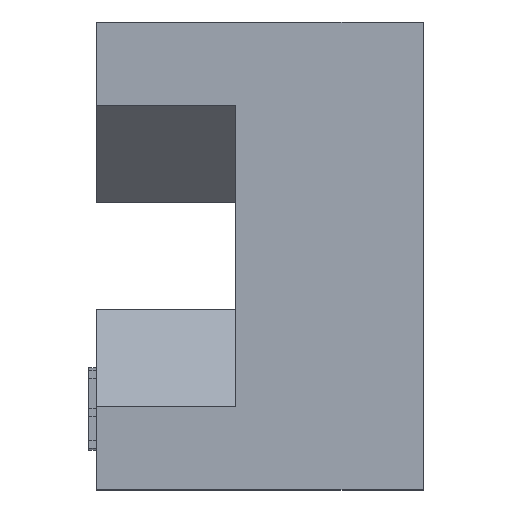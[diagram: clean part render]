
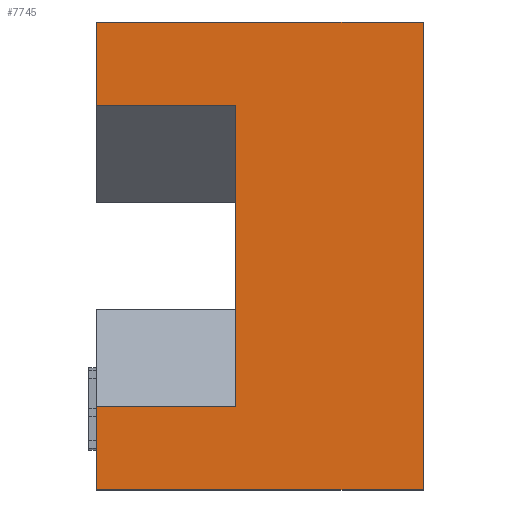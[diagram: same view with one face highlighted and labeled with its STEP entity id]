
A CAD part, left-side view. The second image highlights one B-rep face of the part: STEP entity #7745.
In plain terms, the highlighted planar face has unit normal (-1, 0, 0).
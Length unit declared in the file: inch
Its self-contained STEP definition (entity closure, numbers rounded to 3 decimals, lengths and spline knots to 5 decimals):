
#211 = AXIS2_PLACEMENT_3D ( 'NONE', #12093, #2057, #12024 ) ;
#1074 = EDGE_CURVE ( 'NONE', #7358, #13071, #14157, .T. ) ;
#1104 = ORIENTED_EDGE ( 'NONE', *, *, #9814, .T. ) ;
#1933 = EDGE_CURVE ( 'NONE', #3785, #2814, #14161, .T. ) ;
#1956 = LINE ( 'NONE', #5104, #9508 ) ;
#2057 = DIRECTION ( 'NONE',  ( 1., 0., 0. ) ) ;
#2417 = CARTESIAN_POINT ( 'NONE',  ( -5.5, 0.218, -0.156 ) ) ;
#2568 = EDGE_CURVE ( 'NONE', #11443, #11497, #12649, .T. ) ;
#2814 = VERTEX_POINT ( 'NONE', #7056 ) ;
#3128 = VECTOR ( 'NONE', #6913, 39.37008 ) ;
#3159 = CARTESIAN_POINT ( 'NONE',  ( -5.5, 0.218, -0.156 ) ) ;
#3540 = CARTESIAN_POINT ( 'NONE',  ( -5.5, 0.218, 0.156 ) ) ;
#3581 = ORIENTED_EDGE ( 'NONE', *, *, #14495, .F. ) ;
#3651 = VERTEX_POINT ( 'NONE', #12734 ) ;
#3774 = DIRECTION ( 'NONE',  ( 0., 0., 1. ) ) ;
#3785 = VERTEX_POINT ( 'NONE', #10998 ) ;
#4194 = CARTESIAN_POINT ( 'NONE',  ( -5.5, 0., -0.156 ) ) ;
#4259 = DIRECTION ( 'NONE',  ( 0., 0., 1. ) ) ;
#4280 = EDGE_CURVE ( 'NONE', #7358, #3651, #5325, .T. ) ;
#4372 = VECTOR ( 'NONE', #8225, 39.37008 ) ;
#4618 = DIRECTION ( 'NONE',  ( 0., 0., 1. ) ) ;
#4781 = CARTESIAN_POINT ( 'NONE',  ( -5.5, 0.218, -0.156 ) ) ;
#4852 = LINE ( 'NONE', #3540, #4372 ) ;
#5104 = CARTESIAN_POINT ( 'NONE',  ( -5.5, 0.125, 0.1005 ) ) ;
#5325 = LINE ( 'NONE', #9802, #10900 ) ;
#6170 = CARTESIAN_POINT ( 'NONE',  ( -5.5, 0., 0.156 ) ) ;
#6207 = VERTEX_POINT ( 'NONE', #4781 ) ;
#6913 = DIRECTION ( 'NONE',  ( 0., -1., 0. ) ) ;
#7056 = CARTESIAN_POINT ( 'NONE',  ( -5.5, 0.218, 0.156 ) ) ;
#7256 = VECTOR ( 'NONE', #3774, 39.37008 ) ;
#7358 = VERTEX_POINT ( 'NONE', #12957 ) ;
#7540 = PLANE ( 'NONE',  #211 ) ;
#7745 = ADVANCED_FACE ( 'NONE', ( #10997 ), #7540, .F. ) ;
#7877 = ORIENTED_EDGE ( 'NONE', *, *, #2568, .T. ) ;
#7969 = CARTESIAN_POINT ( 'NONE',  ( -5.5, 0.125, 0.1005 ) ) ;
#8021 = ORIENTED_EDGE ( 'NONE', *, *, #11742, .F. ) ;
#8225 = DIRECTION ( 'NONE',  ( 0., -1., 0. ) ) ;
#8371 = VECTOR ( 'NONE', #4618, 39.37008 ) ;
#9508 = VECTOR ( 'NONE', #10756, 39.37008 ) ;
#9514 = EDGE_LOOP ( 'NONE', ( #14418, #11352, #3581, #1104, #7877, #8021, #13651, #13307 ) ) ;
#9802 = CARTESIAN_POINT ( 'NONE',  ( -5.5, 0.125, -0.1005 ) ) ;
#9814 = EDGE_CURVE ( 'NONE', #6207, #11443, #11602, .T. ) ;
#9831 = VECTOR ( 'NONE', #10943, 39.37008 ) ;
#10365 = CARTESIAN_POINT ( 'NONE',  ( -5.5, 0.218, -0.156 ) ) ;
#10756 = DIRECTION ( 'NONE',  ( 0., 1., 0. ) ) ;
#10900 = VECTOR ( 'NONE', #14278, 39.37008 ) ;
#10943 = DIRECTION ( 'NONE',  ( 0., 0., 1. ) ) ;
#10997 = FACE_OUTER_BOUND ( 'NONE', #9514, .T. ) ;
#10998 = CARTESIAN_POINT ( 'NONE',  ( -5.5, 0.218, 0.1005 ) ) ;
#11352 = ORIENTED_EDGE ( 'NONE', *, *, #4280, .T. ) ;
#11443 = VERTEX_POINT ( 'NONE', #4194 ) ;
#11497 = VERTEX_POINT ( 'NONE', #6170 ) ;
#11507 = LINE ( 'NONE', #2417, #8371 ) ;
#11547 = CARTESIAN_POINT ( 'NONE',  ( -5.5, 0., -0.156 ) ) ;
#11602 = LINE ( 'NONE', #10365, #3128 ) ;
#11742 = EDGE_CURVE ( 'NONE', #2814, #11497, #4852, .T. ) ;
#12024 = DIRECTION ( 'NONE',  ( 0., 0., -1. ) ) ;
#12093 = CARTESIAN_POINT ( 'NONE',  ( -5.5, 0.218, -0.156 ) ) ;
#12649 = LINE ( 'NONE', #11547, #7256 ) ;
#12734 = CARTESIAN_POINT ( 'NONE',  ( -5.5, 0.218, -0.1005 ) ) ;
#12790 = VECTOR ( 'NONE', #4259, 39.37008 ) ;
#12957 = CARTESIAN_POINT ( 'NONE',  ( -5.5, 0.125, -0.1005 ) ) ;
#13062 = CARTESIAN_POINT ( 'NONE',  ( -5.5, 0.125, -0.1005 ) ) ;
#13071 = VERTEX_POINT ( 'NONE', #7969 ) ;
#13307 = ORIENTED_EDGE ( 'NONE', *, *, #13621, .F. ) ;
#13621 = EDGE_CURVE ( 'NONE', #13071, #3785, #1956, .T. ) ;
#13651 = ORIENTED_EDGE ( 'NONE', *, *, #1933, .F. ) ;
#14157 = LINE ( 'NONE', #13062, #12790 ) ;
#14161 = LINE ( 'NONE', #3159, #9831 ) ;
#14278 = DIRECTION ( 'NONE',  ( 0., 1., 0. ) ) ;
#14418 = ORIENTED_EDGE ( 'NONE', *, *, #1074, .F. ) ;
#14495 = EDGE_CURVE ( 'NONE', #6207, #3651, #11507, .T. ) ;
